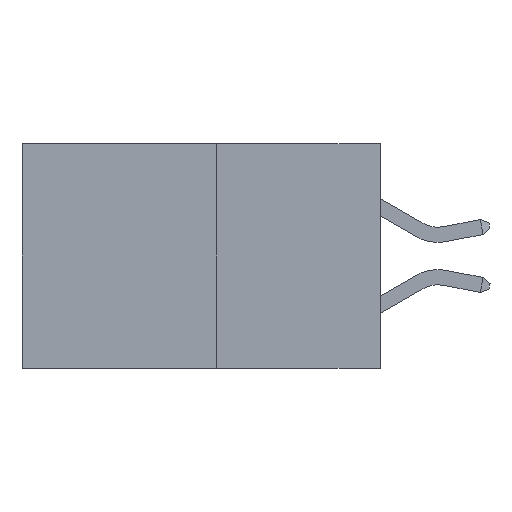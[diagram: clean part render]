
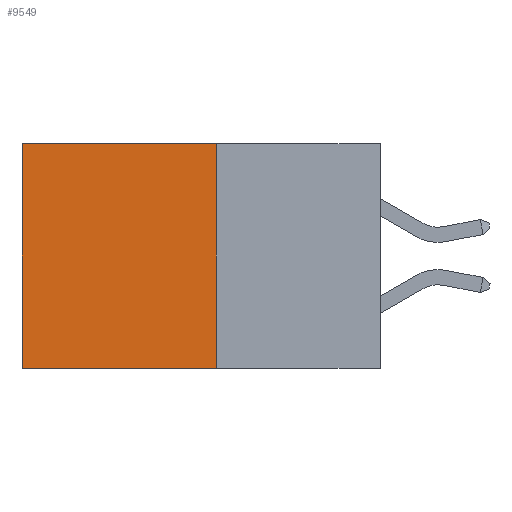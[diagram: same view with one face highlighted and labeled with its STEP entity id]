
A CAD part, left-side view. The second image highlights one B-rep face of the part: STEP entity #9549.
In plain terms, the highlighted planar face has unit normal (-1, 0, 0).
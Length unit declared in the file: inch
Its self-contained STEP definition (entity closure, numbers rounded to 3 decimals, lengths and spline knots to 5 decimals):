
#1083 = ORIENTED_EDGE ( 'NONE', *, *, #7017, .T. ) ;
#1103 = ORIENTED_EDGE ( 'NONE', *, *, #5495, .F. ) ;
#1306 = VECTOR ( 'NONE', #4539, 39.37008 ) ;
#1370 = ORIENTED_EDGE ( 'NONE', *, *, #7649, .F. ) ;
#1512 = ORIENTED_EDGE ( 'NONE', *, *, #4055, .T. ) ;
#1567 = FACE_OUTER_BOUND ( 'NONE', #2410, .T. ) ;
#1667 = LINE ( 'NONE', #9153, #8673 ) ;
#1802 = VECTOR ( 'NONE', #5813, 39.37008 ) ;
#2026 = DIRECTION ( 'NONE',  ( 0., 1., 0. ) ) ;
#2027 = CARTESIAN_POINT ( 'NONE',  ( 0.277, 0.27, -0.37 ) ) ;
#2410 = EDGE_LOOP ( 'NONE', ( #1083, #1103, #1370, #1512 ) ) ;
#2989 = VERTEX_POINT ( 'NONE', #4893 ) ;
#3068 = CARTESIAN_POINT ( 'NONE',  ( 0.277, 0.59, -0.37 ) ) ;
#3130 = CARTESIAN_POINT ( 'NONE',  ( 0.277, 0.59, 0. ) ) ;
#3270 = LINE ( 'NONE', #3068, #1306 ) ;
#3438 = VERTEX_POINT ( 'NONE', #8653 ) ;
#3603 = PLANE ( 'NONE',  #7141 ) ;
#4055 = EDGE_CURVE ( 'NONE', #3438, #7139, #1667, .T. ) ;
#4356 = VERTEX_POINT ( 'NONE', #7328 ) ;
#4539 = DIRECTION ( 'NONE',  ( 0., 0., -1. ) ) ;
#4893 = CARTESIAN_POINT ( 'NONE',  ( 0.277, 0.27, -0.37 ) ) ;
#5061 = CARTESIAN_POINT ( 'NONE',  ( 0.277, 0.27, -0.37 ) ) ;
#5076 = DIRECTION ( 'NONE',  ( 0., 0., -1. ) ) ;
#5243 = LINE ( 'NONE', #2027, #8842 ) ;
#5495 = EDGE_CURVE ( 'NONE', #2989, #4356, #5243, .T. ) ;
#5813 = DIRECTION ( 'NONE',  ( 0., 0., -1. ) ) ;
#7017 = EDGE_CURVE ( 'NONE', #7139, #4356, #3270, .T. ) ;
#7139 = VERTEX_POINT ( 'NONE', #3130 ) ;
#7141 = AXIS2_PLACEMENT_3D ( 'NONE', #8684, #9381, #5076 ) ;
#7328 = CARTESIAN_POINT ( 'NONE',  ( 0.277, 0.59, -0.37 ) ) ;
#7563 = LINE ( 'NONE', #5061, #1802 ) ;
#7649 = EDGE_CURVE ( 'NONE', #3438, #2989, #7563, .T. ) ;
#8653 = CARTESIAN_POINT ( 'NONE',  ( 0.277, 0.27, 0. ) ) ;
#8673 = VECTOR ( 'NONE', #9122, 39.37008 ) ;
#8684 = CARTESIAN_POINT ( 'NONE',  ( 0.277, 0.27, -0.37 ) ) ;
#8842 = VECTOR ( 'NONE', #2026, 39.37008 ) ;
#9122 = DIRECTION ( 'NONE',  ( 0., 1., 0. ) ) ;
#9153 = CARTESIAN_POINT ( 'NONE',  ( 0.277, 0.27, 0. ) ) ;
#9381 = DIRECTION ( 'NONE',  ( 1., 0., 0. ) ) ;
#9549 = ADVANCED_FACE ( 'NONE', ( #1567 ), #3603, .F. ) ;
